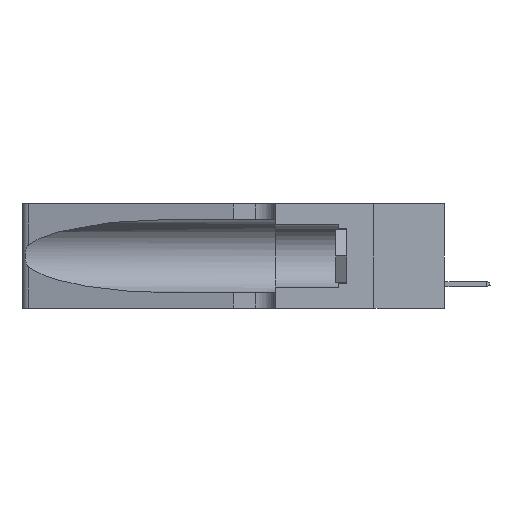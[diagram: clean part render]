
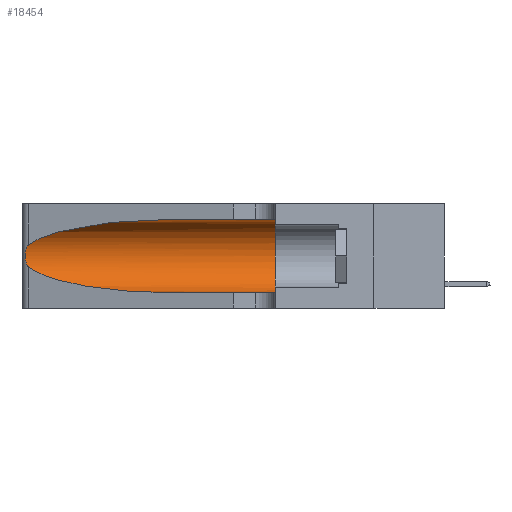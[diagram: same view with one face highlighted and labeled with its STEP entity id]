
A CAD part, left-side view. The second image highlights one B-rep face of the part: STEP entity #18454.
In plain terms, the highlighted cylindrical face has radius 3.308 mm (diameter 6.617 mm), a partial arc.
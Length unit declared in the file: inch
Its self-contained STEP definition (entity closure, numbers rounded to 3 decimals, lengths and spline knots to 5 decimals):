
#363 = CARTESIAN_POINT ( 'NONE',  ( 0.25854, 1.2359, 0.20912 ) ) ;
#494 = CARTESIAN_POINT ( 'NONE',  ( 0.25639, 1.23186, 0.15144 ) ) ;
#886 = DIRECTION ( 'NONE',  ( 0., -1., 0. ) ) ;
#1654 = EDGE_CURVE ( 'NONE', #5999, #36883, #2957, .T. ) ;
#1829 = LINE ( 'NONE', #5605, #28569 ) ;
#2269 = DIRECTION ( 'NONE',  ( 0., 0., 1. ) ) ;
#2957 = LINE ( 'NONE', #21385, #21333 ) ;
#3367 = CARTESIAN_POINT ( 'NONE',  ( 0.2373, 1.15595, 0.08982 ) ) ;
#3639 = CARTESIAN_POINT ( 'NONE',  ( 0.25487, 1.22718, 0.14631 ) ) ;
#4536 = B_SPLINE_CURVE_WITH_KNOTS ( 'NONE', 3,
 ( #6505, #18297, #33315, #6890, #363, #18167, #6391, #9304, #30129, #6622, #29866, #494, #21243, #3639 ),
 .UNSPECIFIED., .F., .F.,
 ( 4, 2, 2, 2, 2, 2, 4 ),
 ( 0., 0.00027, 0.00053, 0.00107, 0.0016, 0.00187, 0.00214 ),
 .UNSPECIFIED. ) ;
#5456 = EDGE_CURVE ( 'NONE', #7156, #32575, #4536, .T. ) ;
#5518 = CARTESIAN_POINT ( 'NONE',  ( 0.1305, 0.35, 0.31525 ) ) ;
#5605 = CARTESIAN_POINT ( 'NONE',  ( 0.1305, 1.61858, 0.31525 ) ) ;
#5999 = VERTEX_POINT ( 'NONE', #27135 ) ;
#6391 = CARTESIAN_POINT ( 'NONE',  ( 0.26075, 1.23896, 0.19203 ) ) ;
#6505 = CARTESIAN_POINT ( 'NONE',  ( 0.25487, 1.22718, 0.22369 ) ) ;
#6622 = CARTESIAN_POINT ( 'NONE',  ( 0.25856, 1.23593, 0.16098 ) ) ;
#6873 = CARTESIAN_POINT ( 'NONE',  ( 0.1305, 0.72297, 0.05475 ) ) ;
#6890 = CARTESIAN_POINT ( 'NONE',  ( 0.25787, 1.23484, 0.2124 ) ) ;
#7156 = VERTEX_POINT ( 'NONE', #37523 ) ;
#7998 = DIRECTION ( 'NONE',  ( 0., 1., 0. ) ) ;
#8646 =( BOUNDED_CURVE ( )  B_SPLINE_CURVE ( 3, ( #24163, #27107, #15636, #33381 ),
 .UNSPECIFIED., .F., .T. ) 
 B_SPLINE_CURVE_WITH_KNOTS ( ( 4, 4 ),
 ( 1.5708, 2.84003 ),
 .UNSPECIFIED. ) 
 CURVE ( )  GEOMETRIC_REPRESENTATION_ITEM ( )  RATIONAL_B_SPLINE_CURVE ( ( 1., 0.87, 0.87, 1. ) ) 
 REPRESENTATION_ITEM ( '' )  );
#9080 = CYLINDRICAL_SURFACE ( 'NONE', #19877, 0.13025 ) ;
#9304 = CARTESIAN_POINT ( 'NONE',  ( 0.26075, 1.23896, 0.178 ) ) ;
#9818 = ORIENTED_EDGE ( 'NONE', *, *, #26602, .T. ) ;
#10771 = CARTESIAN_POINT ( 'NONE',  ( 0.1305, 0.35, 0.185 ) ) ;
#11748 = ORIENTED_EDGE ( 'NONE', *, *, #5456, .T. ) ;
#12729 = FACE_OUTER_BOUND ( 'NONE', #28155, .T. ) ;
#15636 = CARTESIAN_POINT ( 'NONE',  ( 0.2373, 1.15595, 0.28018 ) ) ;
#15716 = CARTESIAN_POINT ( 'NONE',  ( 0.1305, 1.61858, 0.185 ) ) ;
#16570 = ORIENTED_EDGE ( 'NONE', *, *, #1654, .T. ) ;
#16771 = EDGE_CURVE ( 'NONE', #24099, #7156, #8646, .T. ) ;
#17106 =( BOUNDED_CURVE ( )  B_SPLINE_CURVE ( 3, ( #32685, #3367, #30254, #6873 ),
 .UNSPECIFIED., .F., .T. ) 
 B_SPLINE_CURVE_WITH_KNOTS ( ( 4, 4 ),
 ( 3.44316, 4.71239 ),
 .UNSPECIFIED. ) 
 CURVE ( )  GEOMETRIC_REPRESENTATION_ITEM ( )  RATIONAL_B_SPLINE_CURVE ( ( 1., 0.87, 0.87, 1. ) ) 
 REPRESENTATION_ITEM ( '' )  );
#17501 = DIRECTION ( 'NONE',  ( 0., -1., 0. ) ) ;
#18167 = CARTESIAN_POINT ( 'NONE',  ( 0.26018, 1.23835, 0.19895 ) ) ;
#18297 = CARTESIAN_POINT ( 'NONE',  ( 0.25555, 1.22994, 0.2215 ) ) ;
#18454 = ADVANCED_FACE ( 'NONE', ( #12729 ), #9080, .F. ) ;
#19877 = AXIS2_PLACEMENT_3D ( 'NONE', #15716, #30401, #36333 ) ;
#20444 = VERTEX_POINT ( 'NONE', #5518 ) ;
#21243 = CARTESIAN_POINT ( 'NONE',  ( 0.25555, 1.22993, 0.14849 ) ) ;
#21333 = VECTOR ( 'NONE', #886, 39.37008 ) ;
#21385 = CARTESIAN_POINT ( 'NONE',  ( 0.1305, 1.61858, 0.05475 ) ) ;
#21911 = CARTESIAN_POINT ( 'NONE',  ( 0.1305, 0.72297, 0.31525 ) ) ;
#24099 = VERTEX_POINT ( 'NONE', #21911 ) ;
#24163 = CARTESIAN_POINT ( 'NONE',  ( 0.1305, 0.72297, 0.31525 ) ) ;
#25967 = ORIENTED_EDGE ( 'NONE', *, *, #16771, .T. ) ;
#26602 = EDGE_CURVE ( 'NONE', #32575, #5999, #17106, .T. ) ;
#27107 = CARTESIAN_POINT ( 'NONE',  ( 0.18966, 0.96281, 0.31525 ) ) ;
#27135 = CARTESIAN_POINT ( 'NONE',  ( 0.1305, 0.72297, 0.05475 ) ) ;
#28155 = EDGE_LOOP ( 'NONE', ( #25967, #11748, #9818, #16570, #31264, #33941 ) ) ;
#28569 = VECTOR ( 'NONE', #17501, 39.37008 ) ;
#28705 = CIRCLE ( 'NONE', #33873, 0.13025 ) ;
#29866 = CARTESIAN_POINT ( 'NONE',  ( 0.25789, 1.23486, 0.15765 ) ) ;
#30129 = CARTESIAN_POINT ( 'NONE',  ( 0.26017, 1.23833, 0.17102 ) ) ;
#30254 = CARTESIAN_POINT ( 'NONE',  ( 0.18966, 0.96281, 0.05475 ) ) ;
#30401 = DIRECTION ( 'NONE',  ( 0., -1., 0. ) ) ;
#31264 = ORIENTED_EDGE ( 'NONE', *, *, #36780, .F. ) ;
#32575 = VERTEX_POINT ( 'NONE', #36652 ) ;
#32685 = CARTESIAN_POINT ( 'NONE',  ( 0.25487, 1.22718, 0.14631 ) ) ;
#32750 = EDGE_CURVE ( 'NONE', #24099, #20444, #1829, .T. ) ;
#33315 = CARTESIAN_POINT ( 'NONE',  ( 0.25639, 1.23184, 0.21858 ) ) ;
#33381 = CARTESIAN_POINT ( 'NONE',  ( 0.25487, 1.22718, 0.22369 ) ) ;
#33873 = AXIS2_PLACEMENT_3D ( 'NONE', #10771, #7998, #2269 ) ;
#33941 = ORIENTED_EDGE ( 'NONE', *, *, #32750, .F. ) ;
#36333 = DIRECTION ( 'NONE',  ( 0., 0., -1. ) ) ;
#36652 = CARTESIAN_POINT ( 'NONE',  ( 0.25487, 1.22718, 0.14631 ) ) ;
#36780 = EDGE_CURVE ( 'NONE', #20444, #36883, #28705, .T. ) ;
#36883 = VERTEX_POINT ( 'NONE', #37830 ) ;
#37523 = CARTESIAN_POINT ( 'NONE',  ( 0.25487, 1.22718, 0.22369 ) ) ;
#37830 = CARTESIAN_POINT ( 'NONE',  ( 0.1305, 0.35, 0.05475 ) ) ;
